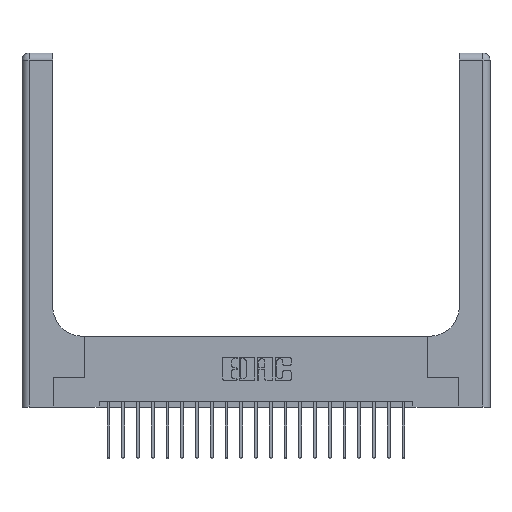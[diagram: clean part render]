
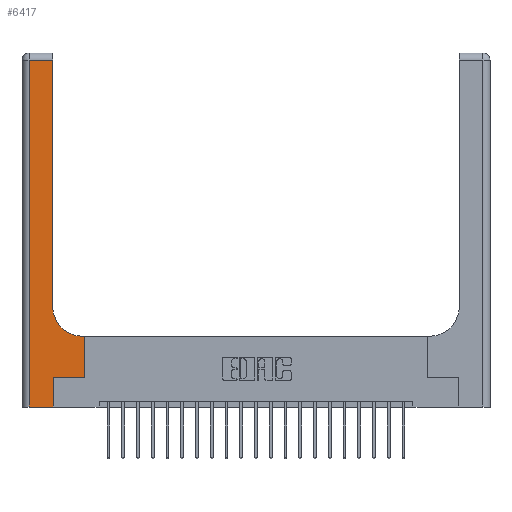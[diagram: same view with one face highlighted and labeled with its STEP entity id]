
A CAD part, top view. The second image highlights one B-rep face of the part: STEP entity #6417.
In plain terms, the highlighted planar face has unit normal (0, 0, 1).
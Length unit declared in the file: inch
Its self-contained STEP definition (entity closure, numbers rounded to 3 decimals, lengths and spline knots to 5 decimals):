
#289 = VECTOR ( 'NONE', #3793, 39.37008 ) ;
#722 = EDGE_LOOP ( 'NONE', ( #15566, #21618, #14473, #21265, #4588, #10088, #9582, #9528, #2761 ) ) ;
#1273 = LINE ( 'NONE', #8138, #17987 ) ;
#1307 = DIRECTION ( 'NONE',  ( 0., 0., -1. ) ) ;
#1440 = CARTESIAN_POINT ( 'NONE',  ( 0., 0., 0.37 ) ) ;
#1590 = LINE ( 'NONE', #13807, #15709 ) ;
#2436 = CARTESIAN_POINT ( 'NONE',  ( 0.51, 0.6, 0.37 ) ) ;
#2619 = CARTESIAN_POINT ( 'NONE',  ( 0.51, 0.85, 0.37 ) ) ;
#2761 = ORIENTED_EDGE ( 'NONE', *, *, #5650, .T. ) ;
#2791 = PLANE ( 'NONE',  #4664 ) ;
#3649 = LINE ( 'NONE', #3870, #4979 ) ;
#3793 = DIRECTION ( 'NONE',  ( 0., -1., 0. ) ) ;
#3870 = CARTESIAN_POINT ( 'NONE',  ( 0., 2.94, 0.37 ) ) ;
#3902 = LINE ( 'NONE', #5477, #289 ) ;
#3979 = DIRECTION ( 'NONE',  ( 1., 0., 0. ) ) ;
#4384 = AXIS2_PLACEMENT_3D ( 'NONE', #2619, #18060, #4510 ) ;
#4510 = DIRECTION ( 'NONE',  ( 1., 0., 0. ) ) ;
#4553 = VERTEX_POINT ( 'NONE', #11810 ) ;
#4588 = ORIENTED_EDGE ( 'NONE', *, *, #22106, .T. ) ;
#4605 = VERTEX_POINT ( 'NONE', #16827 ) ;
#4664 = AXIS2_PLACEMENT_3D ( 'NONE', #16471, #1307, #20259 ) ;
#4979 = VECTOR ( 'NONE', #5780, 39.37008 ) ;
#5049 = VERTEX_POINT ( 'NONE', #7065 ) ;
#5141 = VERTEX_POINT ( 'NONE', #9706 ) ;
#5477 = CARTESIAN_POINT ( 'NONE',  ( 0.06, 3., 0.37 ) ) ;
#5650 = EDGE_CURVE ( 'NONE', #17250, #18480, #14069, .T. ) ;
#5780 = DIRECTION ( 'NONE',  ( -1., 0., 0. ) ) ;
#6371 = FACE_OUTER_BOUND ( 'NONE', #722, .T. ) ;
#6417 = ADVANCED_FACE ( 'NONE', ( #6371 ), #2791, .F. ) ;
#7065 = CARTESIAN_POINT ( 'NONE',  ( 0.265, 0.25, 0.37 ) ) ;
#7773 = VECTOR ( 'NONE', #15397, 39.37008 ) ;
#7812 = LINE ( 'NONE', #18197, #8632 ) ;
#8031 = EDGE_CURVE ( 'NONE', #5049, #5141, #15767, .T. ) ;
#8110 = EDGE_CURVE ( 'NONE', #12190, #10008, #3649, .T. ) ;
#8138 = CARTESIAN_POINT ( 'NONE',  ( 0.26, 3., 0.37 ) ) ;
#8632 = VECTOR ( 'NONE', #21573, 39.37008 ) ;
#8942 = CARTESIAN_POINT ( 'NONE',  ( 0.265, 0.25, 0.37 ) ) ;
#9106 = CARTESIAN_POINT ( 'NONE',  ( 0.265, 0., 0.37 ) ) ;
#9528 = ORIENTED_EDGE ( 'NONE', *, *, #19784, .T. ) ;
#9582 = ORIENTED_EDGE ( 'NONE', *, *, #17910, .T. ) ;
#9706 = CARTESIAN_POINT ( 'NONE',  ( 0.528, 0.25, 0.37 ) ) ;
#10008 = VERTEX_POINT ( 'NONE', #13270 ) ;
#10088 = ORIENTED_EDGE ( 'NONE', *, *, #8031, .T. ) ;
#10726 = EDGE_CURVE ( 'NONE', #18480, #12190, #1273, .T. ) ;
#11777 = DIRECTION ( 'NONE',  ( 1., 0., 0. ) ) ;
#11810 = CARTESIAN_POINT ( 'NONE',  ( 0.06, 0., 0.37 ) ) ;
#11847 = EDGE_CURVE ( 'NONE', #4553, #15870, #16902, .T. ) ;
#12142 = VECTOR ( 'NONE', #3979, 39.37008 ) ;
#12190 = VERTEX_POINT ( 'NONE', #21488 ) ;
#13270 = CARTESIAN_POINT ( 'NONE',  ( 0.06, 2.94, 0.37 ) ) ;
#13807 = CARTESIAN_POINT ( 'NONE',  ( 0.26, 0.6, 0.37 ) ) ;
#14069 = CIRCLE ( 'NONE', #4384, 0.25 ) ;
#14378 = CARTESIAN_POINT ( 'NONE',  ( 0.26, 0.85, 0.37 ) ) ;
#14473 = ORIENTED_EDGE ( 'NONE', *, *, #20348, .T. ) ;
#15172 = CARTESIAN_POINT ( 'NONE',  ( 0.528, 0.25, 0.37 ) ) ;
#15397 = DIRECTION ( 'NONE',  ( 0., 1., 0. ) ) ;
#15566 = ORIENTED_EDGE ( 'NONE', *, *, #10726, .T. ) ;
#15709 = VECTOR ( 'NONE', #20647, 39.37008 ) ;
#15767 = LINE ( 'NONE', #8942, #12142 ) ;
#15870 = VERTEX_POINT ( 'NONE', #9106 ) ;
#16227 = VECTOR ( 'NONE', #11777, 39.37008 ) ;
#16471 = CARTESIAN_POINT ( 'NONE',  ( 0., 3., 0.37 ) ) ;
#16827 = CARTESIAN_POINT ( 'NONE',  ( 0.528, 0.6, 0.37 ) ) ;
#16902 = LINE ( 'NONE', #1440, #16227 ) ;
#17250 = VERTEX_POINT ( 'NONE', #2436 ) ;
#17910 = EDGE_CURVE ( 'NONE', #5141, #4605, #18740, .T. ) ;
#17987 = VECTOR ( 'NONE', #20344, 39.37008 ) ;
#18060 = DIRECTION ( 'NONE',  ( 0., 0., -1. ) ) ;
#18197 = CARTESIAN_POINT ( 'NONE',  ( 0.265, 0., 0.37 ) ) ;
#18480 = VERTEX_POINT ( 'NONE', #14378 ) ;
#18740 = LINE ( 'NONE', #15172, #7773 ) ;
#19784 = EDGE_CURVE ( 'NONE', #4605, #17250, #1590, .T. ) ;
#20259 = DIRECTION ( 'NONE',  ( -1., 0., 0. ) ) ;
#20344 = DIRECTION ( 'NONE',  ( 0., 1., 0. ) ) ;
#20348 = EDGE_CURVE ( 'NONE', #10008, #4553, #3902, .T. ) ;
#20647 = DIRECTION ( 'NONE',  ( -1., 0., 0. ) ) ;
#21265 = ORIENTED_EDGE ( 'NONE', *, *, #11847, .T. ) ;
#21488 = CARTESIAN_POINT ( 'NONE',  ( 0.26, 2.94, 0.37 ) ) ;
#21573 = DIRECTION ( 'NONE',  ( 0., 1., 0. ) ) ;
#21618 = ORIENTED_EDGE ( 'NONE', *, *, #8110, .T. ) ;
#22106 = EDGE_CURVE ( 'NONE', #15870, #5049, #7812, .T. ) ;
